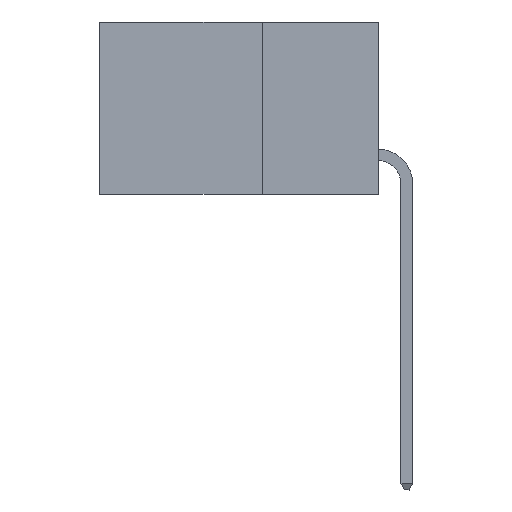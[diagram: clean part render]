
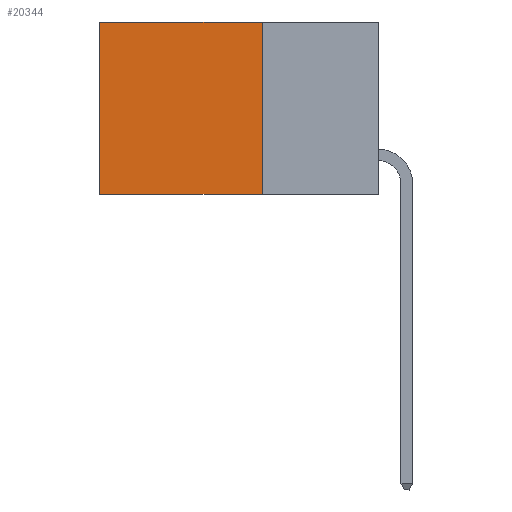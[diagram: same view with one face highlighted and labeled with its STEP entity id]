
A CAD part, left-side view. The second image highlights one B-rep face of the part: STEP entity #20344.
In plain terms, the highlighted planar face has unit normal (-1, 0, 0).
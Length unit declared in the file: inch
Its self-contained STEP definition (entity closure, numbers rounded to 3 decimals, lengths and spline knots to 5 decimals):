
#800 = DIRECTION ( 'NONE',  ( 0., 1., 0. ) ) ;
#1412 = DIRECTION ( 'NONE',  ( 0., 1., 0. ) ) ;
#1818 = EDGE_CURVE ( 'NONE', #12787, #3946, #15766, .T. ) ;
#2793 = CARTESIAN_POINT ( 'NONE',  ( 0.2615, 0.25, -0.37 ) ) ;
#2810 = VERTEX_POINT ( 'NONE', #18066 ) ;
#3141 = DIRECTION ( 'NONE',  ( 1., 0., 0. ) ) ;
#3285 = EDGE_LOOP ( 'NONE', ( #4209, #16987, #7648, #9076 ) ) ;
#3946 = VERTEX_POINT ( 'NONE', #21808 ) ;
#4209 = ORIENTED_EDGE ( 'NONE', *, *, #20203, .T. ) ;
#4932 = CARTESIAN_POINT ( 'NONE',  ( 0.2615, 0.6, 0. ) ) ;
#5027 = VECTOR ( 'NONE', #17239, 39.37008 ) ;
#6887 = FACE_OUTER_BOUND ( 'NONE', #3285, .T. ) ;
#7608 = VERTEX_POINT ( 'NONE', #4932 ) ;
#7648 = ORIENTED_EDGE ( 'NONE', *, *, #13741, .F. ) ;
#7804 = AXIS2_PLACEMENT_3D ( 'NONE', #8189, #3141, #19438 ) ;
#8189 = CARTESIAN_POINT ( 'NONE',  ( 0.2615, 0.25, -0.37 ) ) ;
#9076 = ORIENTED_EDGE ( 'NONE', *, *, #19448, .T. ) ;
#9314 = VECTOR ( 'NONE', #11288, 39.37008 ) ;
#10086 = PLANE ( 'NONE',  #7804 ) ;
#11288 = DIRECTION ( 'NONE',  ( 0., 0., -1. ) ) ;
#12266 = LINE ( 'NONE', #17468, #16463 ) ;
#12787 = VERTEX_POINT ( 'NONE', #2793 ) ;
#13741 = EDGE_CURVE ( 'NONE', #2810, #12787, #17597, .T. ) ;
#13912 = VECTOR ( 'NONE', #800, 39.37008 ) ;
#14823 = LINE ( 'NONE', #22059, #9314 ) ;
#15766 = LINE ( 'NONE', #22980, #13912 ) ;
#16463 = VECTOR ( 'NONE', #1412, 39.37008 ) ;
#16987 = ORIENTED_EDGE ( 'NONE', *, *, #1818, .F. ) ;
#17239 = DIRECTION ( 'NONE',  ( 0., 0., -1. ) ) ;
#17468 = CARTESIAN_POINT ( 'NONE',  ( 0.2615, 0.25, 0. ) ) ;
#17597 = LINE ( 'NONE', #22694, #5027 ) ;
#18066 = CARTESIAN_POINT ( 'NONE',  ( 0.2615, 0.25, 0. ) ) ;
#19438 = DIRECTION ( 'NONE',  ( 0., 0., -1. ) ) ;
#19448 = EDGE_CURVE ( 'NONE', #2810, #7608, #12266, .T. ) ;
#20203 = EDGE_CURVE ( 'NONE', #7608, #3946, #14823, .T. ) ;
#20344 = ADVANCED_FACE ( 'NONE', ( #6887 ), #10086, .F. ) ;
#21808 = CARTESIAN_POINT ( 'NONE',  ( 0.2615, 0.6, -0.37 ) ) ;
#22059 = CARTESIAN_POINT ( 'NONE',  ( 0.2615, 0.6, -0.37 ) ) ;
#22694 = CARTESIAN_POINT ( 'NONE',  ( 0.2615, 0.25, -0.37 ) ) ;
#22980 = CARTESIAN_POINT ( 'NONE',  ( 0.2615, 0.25, -0.37 ) ) ;
